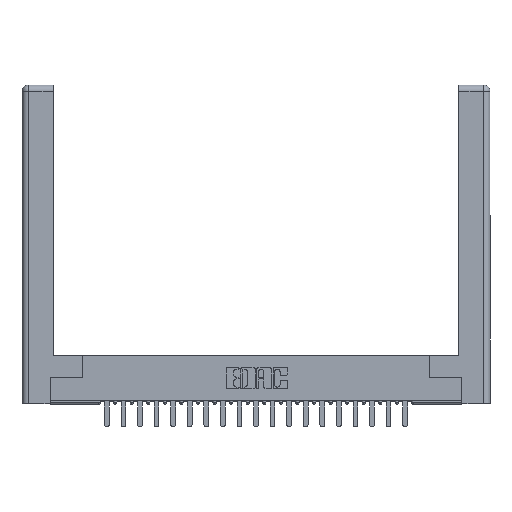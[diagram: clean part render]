
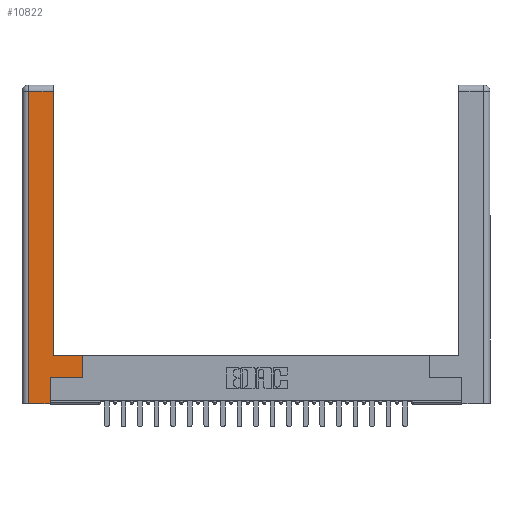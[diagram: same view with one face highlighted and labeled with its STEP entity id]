
A CAD part, top view. The second image highlights one B-rep face of the part: STEP entity #10822.
In plain terms, the highlighted planar face has unit normal (0, 0, 1).
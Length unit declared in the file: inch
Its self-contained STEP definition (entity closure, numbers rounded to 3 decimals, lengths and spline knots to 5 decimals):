
#205 = EDGE_CURVE ( 'NONE', #16018, #11239, #4804, .T. ) ;
#1604 = LINE ( 'NONE', #10252, #12885 ) ;
#1803 = EDGE_CURVE ( 'NONE', #5583, #4200, #11284, .T. ) ;
#1969 = AXIS2_PLACEMENT_3D ( 'NONE', #23750, #15604, #25010 ) ;
#2500 = CARTESIAN_POINT ( 'NONE',  ( 0.295, 0.45, 0. ) ) ;
#2801 = ORIENTED_EDGE ( 'NONE', *, *, #13306, .T. ) ;
#3510 = DIRECTION ( 'NONE',  ( 0., -1., 0. ) ) ;
#3567 = VECTOR ( 'NONE', #6605, 39.37008 ) ;
#3613 = DIRECTION ( 'NONE',  ( 0., 1., 0. ) ) ;
#3620 = ORIENTED_EDGE ( 'NONE', *, *, #23024, .T. ) ;
#4134 = VECTOR ( 'NONE', #15755, 39.37008 ) ;
#4200 = VERTEX_POINT ( 'NONE', #20630 ) ;
#4804 = LINE ( 'NONE', #14874, #16718 ) ;
#5353 = ORIENTED_EDGE ( 'NONE', *, *, #205, .T. ) ;
#5583 = VERTEX_POINT ( 'NONE', #23588 ) ;
#6212 = CARTESIAN_POINT ( 'NONE',  ( 0.265, 0., 0. ) ) ;
#6605 = DIRECTION ( 'NONE',  ( -1., 0., 0. ) ) ;
#6768 = CARTESIAN_POINT ( 'NONE',  ( 0.295, 2.94, 0. ) ) ;
#6972 = DIRECTION ( 'NONE',  ( 1., 0., 0. ) ) ;
#7180 = EDGE_CURVE ( 'NONE', #13874, #7579, #11331, .T. ) ;
#7579 = VERTEX_POINT ( 'NONE', #6212 ) ;
#7798 = ORIENTED_EDGE ( 'NONE', *, *, #7180, .T. ) ;
#8893 = VERTEX_POINT ( 'NONE', #6768 ) ;
#9543 = CARTESIAN_POINT ( 'NONE',  ( 0.565, 0.245, 0. ) ) ;
#9757 = PLANE ( 'NONE',  #1969 ) ;
#9909 = DIRECTION ( 'NONE',  ( 0., 1., 0. ) ) ;
#10066 = EDGE_CURVE ( 'NONE', #8893, #11565, #12073, .T. ) ;
#10157 = LINE ( 'NONE', #15607, #19183 ) ;
#10252 = CARTESIAN_POINT ( 'NONE',  ( 0.265, 0.245, 0. ) ) ;
#10822 = ADVANCED_FACE ( 'NONE', ( #11059 ), #9757, .F. ) ;
#10937 = VECTOR ( 'NONE', #3510, 39.37008 ) ;
#11059 = FACE_OUTER_BOUND ( 'NONE', #16924, .T. ) ;
#11239 = VERTEX_POINT ( 'NONE', #9543 ) ;
#11284 = LINE ( 'NONE', #2500, #12247 ) ;
#11331 = LINE ( 'NONE', #25790, #4134 ) ;
#11565 = VERTEX_POINT ( 'NONE', #24670 ) ;
#12073 = LINE ( 'NONE', #20625, #3567 ) ;
#12247 = VECTOR ( 'NONE', #12375, 39.37008 ) ;
#12375 = DIRECTION ( 'NONE',  ( -1., 0., 0. ) ) ;
#12885 = VECTOR ( 'NONE', #14273, 39.37008 ) ;
#13124 = LINE ( 'NONE', #21703, #10937 ) ;
#13306 = EDGE_CURVE ( 'NONE', #11565, #13874, #13124, .T. ) ;
#13874 = VERTEX_POINT ( 'NONE', #25660 ) ;
#13922 = EDGE_CURVE ( 'NONE', #4200, #8893, #19335, .T. ) ;
#14037 = VECTOR ( 'NONE', #9909, 39.37008 ) ;
#14273 = DIRECTION ( 'NONE',  ( 0., 1., 0. ) ) ;
#14874 = CARTESIAN_POINT ( 'NONE',  ( 0.565, 0.245, 0. ) ) ;
#15604 = DIRECTION ( 'NONE',  ( 0., 0., -1. ) ) ;
#15607 = CARTESIAN_POINT ( 'NONE',  ( 0.565, 0.45, 0. ) ) ;
#15755 = DIRECTION ( 'NONE',  ( 1., 0., 0. ) ) ;
#16018 = VERTEX_POINT ( 'NONE', #24184 ) ;
#16718 = VECTOR ( 'NONE', #6972, 39.37008 ) ;
#16783 = ORIENTED_EDGE ( 'NONE', *, *, #24540, .T. ) ;
#16924 = EDGE_LOOP ( 'NONE', ( #19022, #24936, #2801, #7798, #16783, #5353, #3620, #20420 ) ) ;
#18075 = CARTESIAN_POINT ( 'NONE',  ( 0.295, 3., 0. ) ) ;
#19022 = ORIENTED_EDGE ( 'NONE', *, *, #13922, .T. ) ;
#19183 = VECTOR ( 'NONE', #3613, 39.37008 ) ;
#19335 = LINE ( 'NONE', #18075, #14037 ) ;
#20420 = ORIENTED_EDGE ( 'NONE', *, *, #1803, .T. ) ;
#20625 = CARTESIAN_POINT ( 'NONE',  ( 0.0615, 2.94, 0. ) ) ;
#20630 = CARTESIAN_POINT ( 'NONE',  ( 0.295, 0.45, 0. ) ) ;
#21703 = CARTESIAN_POINT ( 'NONE',  ( 0.0615, 0., 0. ) ) ;
#23024 = EDGE_CURVE ( 'NONE', #11239, #5583, #10157, .T. ) ;
#23588 = CARTESIAN_POINT ( 'NONE',  ( 0.565, 0.45, 0. ) ) ;
#23750 = CARTESIAN_POINT ( 'NONE',  ( 0., 0., 0. ) ) ;
#24184 = CARTESIAN_POINT ( 'NONE',  ( 0.265, 0.245, 0. ) ) ;
#24540 = EDGE_CURVE ( 'NONE', #7579, #16018, #1604, .T. ) ;
#24670 = CARTESIAN_POINT ( 'NONE',  ( 0.0615, 2.94, 0. ) ) ;
#24936 = ORIENTED_EDGE ( 'NONE', *, *, #10066, .T. ) ;
#25010 = DIRECTION ( 'NONE',  ( -1., 0., 0. ) ) ;
#25660 = CARTESIAN_POINT ( 'NONE',  ( 0.0615, 0., 0. ) ) ;
#25790 = CARTESIAN_POINT ( 'NONE',  ( 0.265, 0., 0. ) ) ;
